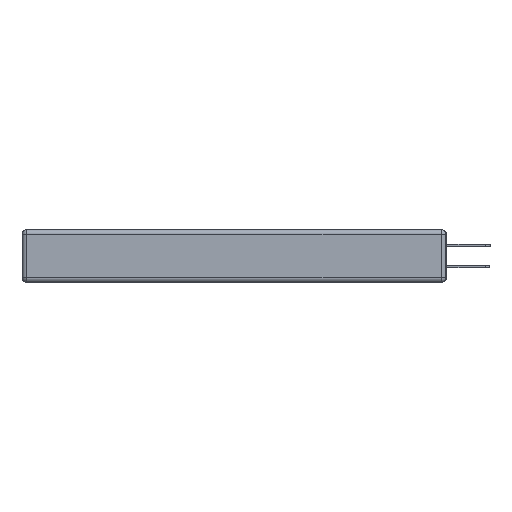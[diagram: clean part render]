
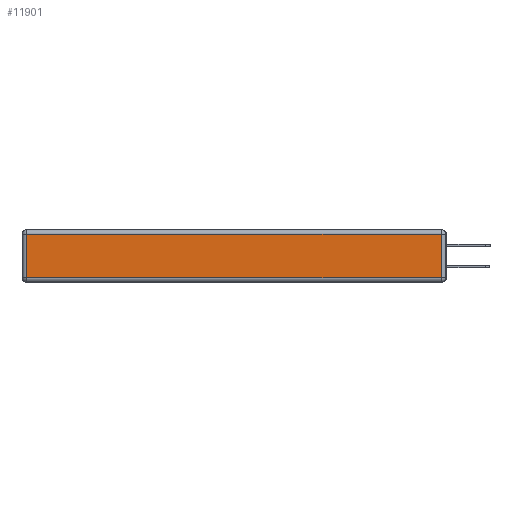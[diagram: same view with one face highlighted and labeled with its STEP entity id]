
A CAD part, left-side view. The second image highlights one B-rep face of the part: STEP entity #11901.
In plain terms, the highlighted planar face has unit normal (-1, 0, 0).
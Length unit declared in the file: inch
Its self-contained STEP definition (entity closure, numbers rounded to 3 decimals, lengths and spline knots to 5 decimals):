
#718 = DIRECTION ( 'NONE',  ( -1., 0., 0. ) ) ;
#805 = DIRECTION ( 'NONE',  ( 0., 0., 1. ) ) ;
#1002 = VECTOR ( 'NONE', #14714, 39.37008 ) ;
#2614 = CARTESIAN_POINT ( 'NONE',  ( 0., 0., -0.343 ) ) ;
#2765 = AXIS2_PLACEMENT_3D ( 'NONE', #2614, #718, #805 ) ;
#3021 = FACE_OUTER_BOUND ( 'NONE', #14247, .T. ) ;
#4290 = ORIENTED_EDGE ( 'NONE', *, *, #20293, .T. ) ;
#4444 = DIRECTION ( 'NONE',  ( 0., 1., 0. ) ) ;
#4814 = ORIENTED_EDGE ( 'NONE', *, *, #5385, .T. ) ;
#5385 = EDGE_CURVE ( 'NONE', #8875, #8528, #16476, .T. ) ;
#8528 = VERTEX_POINT ( 'NONE', #17761 ) ;
#8687 = CARTESIAN_POINT ( 'NONE',  ( 0., 2.75, -0.03 ) ) ;
#8875 = VERTEX_POINT ( 'NONE', #10980 ) ;
#9460 = VERTEX_POINT ( 'NONE', #24534 ) ;
#9470 = EDGE_CURVE ( 'NONE', #16807, #8875, #10455, .T. ) ;
#9685 = EDGE_CURVE ( 'NONE', #9460, #16807, #16762, .T. ) ;
#10455 = LINE ( 'NONE', #20447, #13766 ) ;
#10980 = CARTESIAN_POINT ( 'NONE',  ( 0., 0.03, -0.313 ) ) ;
#10984 = DIRECTION ( 'NONE',  ( 0., 0., 1. ) ) ;
#11298 = CARTESIAN_POINT ( 'NONE',  ( 0., 2.72, -0.313 ) ) ;
#11768 = VECTOR ( 'NONE', #4444, 39.37008 ) ;
#11901 = ADVANCED_FACE ( 'NONE', ( #3021 ), #17981, .T. ) ;
#13766 = VECTOR ( 'NONE', #18855, 39.37008 ) ;
#14247 = EDGE_LOOP ( 'NONE', ( #14382, #4814, #4290, #21237 ) ) ;
#14382 = ORIENTED_EDGE ( 'NONE', *, *, #9470, .T. ) ;
#14551 = CARTESIAN_POINT ( 'NONE',  ( 0., 2.72, -0.343 ) ) ;
#14714 = DIRECTION ( 'NONE',  ( 0., 0., -1. ) ) ;
#16476 = LINE ( 'NONE', #22633, #23845 ) ;
#16762 = LINE ( 'NONE', #14551, #1002 ) ;
#16807 = VERTEX_POINT ( 'NONE', #11298 ) ;
#17761 = CARTESIAN_POINT ( 'NONE',  ( 0., 0.03, -0.03 ) ) ;
#17981 = PLANE ( 'NONE',  #2765 ) ;
#18855 = DIRECTION ( 'NONE',  ( 0., -1., 0. ) ) ;
#19666 = LINE ( 'NONE', #8687, #11768 ) ;
#20293 = EDGE_CURVE ( 'NONE', #8528, #9460, #19666, .T. ) ;
#20447 = CARTESIAN_POINT ( 'NONE',  ( 0., 0., -0.313 ) ) ;
#21237 = ORIENTED_EDGE ( 'NONE', *, *, #9685, .T. ) ;
#22633 = CARTESIAN_POINT ( 'NONE',  ( 0., 0.03, -0.343 ) ) ;
#23845 = VECTOR ( 'NONE', #10984, 39.37008 ) ;
#24534 = CARTESIAN_POINT ( 'NONE',  ( 0., 2.72, -0.03 ) ) ;
